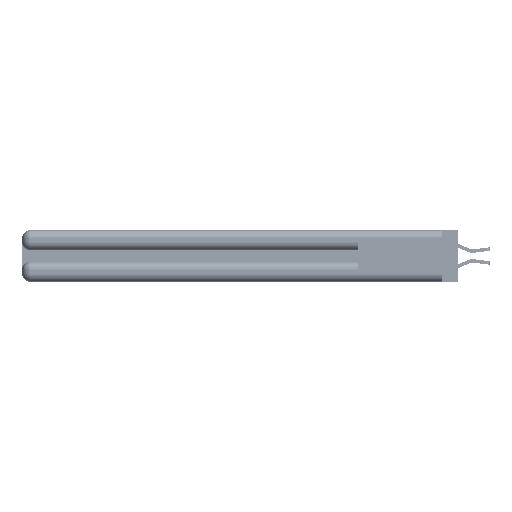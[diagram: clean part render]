
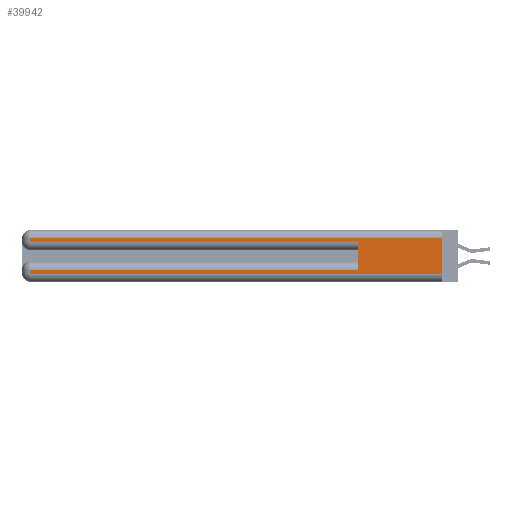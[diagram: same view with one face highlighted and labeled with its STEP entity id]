
A CAD part, left-side view. The second image highlights one B-rep face of the part: STEP entity #39942.
In plain terms, the highlighted planar face has unit normal (-1, 0, 0).
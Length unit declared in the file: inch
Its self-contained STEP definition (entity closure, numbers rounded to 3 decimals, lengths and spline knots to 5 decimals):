
#622 = CARTESIAN_POINT ( 'NONE',  ( 0., 0., 0.285 ) ) ;
#1800 = CARTESIAN_POINT ( 'NONE',  ( 0., 2.94, 0.37 ) ) ;
#2235 = CARTESIAN_POINT ( 'NONE',  ( 0., 0., 0.06 ) ) ;
#2731 = VERTEX_POINT ( 'NONE', #18163 ) ;
#3013 = LINE ( 'NONE', #1800, #44504 ) ;
#4174 = CARTESIAN_POINT ( 'NONE',  ( 0., 0., 0.085 ) ) ;
#5151 = VERTEX_POINT ( 'NONE', #30829 ) ;
#6022 = CARTESIAN_POINT ( 'NONE',  ( 0., 0., 0.06 ) ) ;
#6146 = CARTESIAN_POINT ( 'NONE',  ( 0., 0., 0.31 ) ) ;
#6379 = ORIENTED_EDGE ( 'NONE', *, *, #38556, .T. ) ;
#6697 = CARTESIAN_POINT ( 'NONE',  ( 0., 2.94, 0.37 ) ) ;
#8567 = CARTESIAN_POINT ( 'NONE',  ( 0., 0.6, 0.145 ) ) ;
#9294 = CARTESIAN_POINT ( 'NONE',  ( 0., 2.94, 0.085 ) ) ;
#9589 = VERTEX_POINT ( 'NONE', #6022 ) ;
#10014 = AXIS2_PLACEMENT_3D ( 'NONE', #29274, #21784, #39720 ) ;
#11619 = EDGE_CURVE ( 'NONE', #20916, #2731, #27688, .T. ) ;
#12224 = DIRECTION ( 'NONE',  ( 0., -1., 0. ) ) ;
#14055 = VECTOR ( 'NONE', #46533, 39.37008 ) ;
#14323 = FACE_OUTER_BOUND ( 'NONE', #32962, .T. ) ;
#14398 = EDGE_CURVE ( 'NONE', #42437, #37809, #43421, .T. ) ;
#14558 = VECTOR ( 'NONE', #24671, 39.37008 ) ;
#14582 = EDGE_CURVE ( 'NONE', #37809, #5151, #3013, .T. ) ;
#16515 = VECTOR ( 'NONE', #38259, 39.37008 ) ;
#17358 = CARTESIAN_POINT ( 'NONE',  ( 0., 2.94, 0.285 ) ) ;
#18163 = CARTESIAN_POINT ( 'NONE',  ( 0., 0.6, 0.285 ) ) ;
#19608 = VERTEX_POINT ( 'NONE', #43401 ) ;
#19754 = DIRECTION ( 'NONE',  ( 0., 0., -1. ) ) ;
#20409 = LINE ( 'NONE', #6697, #45432 ) ;
#20539 = ORIENTED_EDGE ( 'NONE', *, *, #11619, .T. ) ;
#20916 = VERTEX_POINT ( 'NONE', #17358 ) ;
#21784 = DIRECTION ( 'NONE',  ( 1., 0., 0. ) ) ;
#22380 = DIRECTION ( 'NONE',  ( 0., 0., -1. ) ) ;
#23269 = ORIENTED_EDGE ( 'NONE', *, *, #31890, .T. ) ;
#23608 = LINE ( 'NONE', #8567, #35521 ) ;
#24076 = ORIENTED_EDGE ( 'NONE', *, *, #14582, .T. ) ;
#24281 = VECTOR ( 'NONE', #12224, 39.37008 ) ;
#24671 = DIRECTION ( 'NONE',  ( 0., -1., 0. ) ) ;
#25984 = EDGE_CURVE ( 'NONE', #42437, #2731, #23608, .T. ) ;
#26236 = LINE ( 'NONE', #38729, #16515 ) ;
#26498 = CARTESIAN_POINT ( 'NONE',  ( 0., 0.6, 0.085 ) ) ;
#27688 = LINE ( 'NONE', #622, #24281 ) ;
#27737 = LINE ( 'NONE', #6146, #14055 ) ;
#28969 = PLANE ( 'NONE',  #10014 ) ;
#29274 = CARTESIAN_POINT ( 'NONE',  ( 0., 0., 0.37 ) ) ;
#30770 = DIRECTION ( 'NONE',  ( 0., 1., 0. ) ) ;
#30829 = CARTESIAN_POINT ( 'NONE',  ( 0., 2.94, 0.06 ) ) ;
#31075 = ORIENTED_EDGE ( 'NONE', *, *, #40386, .F. ) ;
#31890 = EDGE_CURVE ( 'NONE', #19608, #20916, #20409, .T. ) ;
#32072 = VECTOR ( 'NONE', #30770, 39.37008 ) ;
#32962 = EDGE_LOOP ( 'NONE', ( #31075, #6379, #23269, #20539, #42339, #37696, #24076, #43906 ) ) ;
#34034 = DIRECTION ( 'NONE',  ( 0., 0., 1. ) ) ;
#35521 = VECTOR ( 'NONE', #34034, 39.37008 ) ;
#35559 = LINE ( 'NONE', #2235, #14558 ) ;
#37275 = EDGE_CURVE ( 'NONE', #5151, #9589, #35559, .T. ) ;
#37696 = ORIENTED_EDGE ( 'NONE', *, *, #14398, .T. ) ;
#37809 = VERTEX_POINT ( 'NONE', #9294 ) ;
#38259 = DIRECTION ( 'NONE',  ( 0., 0., -1. ) ) ;
#38556 = EDGE_CURVE ( 'NONE', #41665, #19608, #27737, .T. ) ;
#38729 = CARTESIAN_POINT ( 'NONE',  ( 0., 0., 0.37 ) ) ;
#39720 = DIRECTION ( 'NONE',  ( 0., 0., -1. ) ) ;
#39942 = ADVANCED_FACE ( 'NONE', ( #14323 ), #28969, .F. ) ;
#40386 = EDGE_CURVE ( 'NONE', #41665, #9589, #26236, .T. ) ;
#41665 = VERTEX_POINT ( 'NONE', #44146 ) ;
#42339 = ORIENTED_EDGE ( 'NONE', *, *, #25984, .F. ) ;
#42437 = VERTEX_POINT ( 'NONE', #26498 ) ;
#43401 = CARTESIAN_POINT ( 'NONE',  ( 0., 2.94, 0.31 ) ) ;
#43421 = LINE ( 'NONE', #4174, #32072 ) ;
#43906 = ORIENTED_EDGE ( 'NONE', *, *, #37275, .T. ) ;
#44146 = CARTESIAN_POINT ( 'NONE',  ( 0., 0., 0.31 ) ) ;
#44504 = VECTOR ( 'NONE', #19754, 39.37008 ) ;
#45432 = VECTOR ( 'NONE', #22380, 39.37008 ) ;
#46533 = DIRECTION ( 'NONE',  ( 0., 1., 0. ) ) ;
